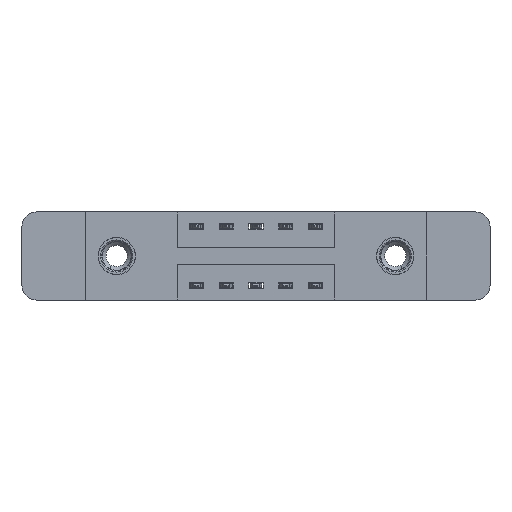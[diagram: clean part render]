
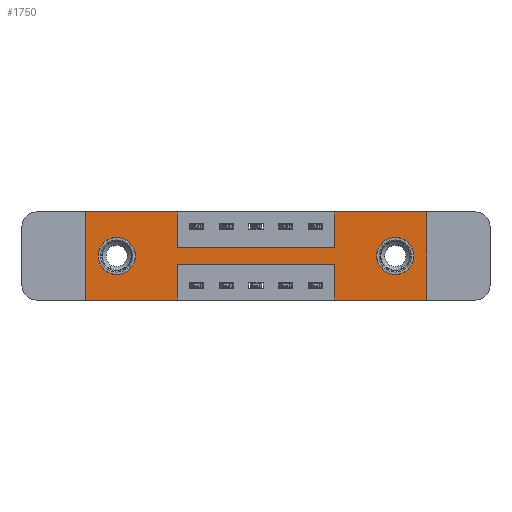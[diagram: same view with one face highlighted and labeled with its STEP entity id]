
A CAD part, front view. The second image highlights one B-rep face of the part: STEP entity #1750.
In plain terms, the highlighted planar face has unit normal (0, -1, 0).
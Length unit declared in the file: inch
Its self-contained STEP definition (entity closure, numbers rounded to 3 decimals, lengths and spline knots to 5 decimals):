
#126 = CIRCLE ( 'NONE', #325, 0.078 ) ;
#208 = DIRECTION ( 'NONE',  ( 0., 0., -1. ) ) ;
#225 = CARTESIAN_POINT ( 'NONE',  ( 0.3875, 0., -0.37 ) ) ;
#251 = DIRECTION ( 'NONE',  ( 0., 1., 0. ) ) ;
#325 = AXIS2_PLACEMENT_3D ( 'NONE', #10204, #13440, #1972 ) ;
#405 = VERTEX_POINT ( 'NONE', #8320 ) ;
#423 = ORIENTED_EDGE ( 'NONE', *, *, #3443, .T. ) ;
#483 = CARTESIAN_POINT ( 'NONE',  ( 0., 0., -0.37 ) ) ;
#484 = LINE ( 'NONE', #9128, #3106 ) ;
#711 = FACE_BOUND ( 'NONE', #7134, .T. ) ;
#802 = VERTEX_POINT ( 'NONE', #5080 ) ;
#832 = DIRECTION ( 'NONE',  ( 0., 0., -1. ) ) ;
#887 = CARTESIAN_POINT ( 'NONE',  ( 0., 0., 0. ) ) ;
#985 = DIRECTION ( 'NONE',  ( -1., 0., 0. ) ) ;
#1118 = VERTEX_POINT ( 'NONE', #9401 ) ;
#1128 = EDGE_CURVE ( 'NONE', #8901, #7750, #3313, .T. ) ;
#1283 = CARTESIAN_POINT ( 'NONE',  ( 0.3875, 0., -0.15 ) ) ;
#1629 = DIRECTION ( 'NONE',  ( 0., 0., 1. ) ) ;
#1730 = CARTESIAN_POINT ( 'NONE',  ( 0.1325, 0., -0.185 ) ) ;
#1750 = ADVANCED_FACE ( 'NONE', ( #4308, #711, #3184 ), #10912, .T. ) ;
#1767 = VERTEX_POINT ( 'NONE', #9796 ) ;
#1933 = EDGE_CURVE ( 'NONE', #405, #2278, #11183, .T. ) ;
#1972 = DIRECTION ( 'NONE',  ( 0., 0., 1. ) ) ;
#1990 = EDGE_CURVE ( 'NONE', #1767, #405, #12183, .T. ) ;
#2102 = DIRECTION ( 'NONE',  ( 1., 0., 0. ) ) ;
#2123 = EDGE_CURVE ( 'NONE', #6096, #5259, #12951, .T. ) ;
#2132 = CARTESIAN_POINT ( 'NONE',  ( 1.3025, 0., -0.263 ) ) ;
#2149 = LINE ( 'NONE', #887, #3919 ) ;
#2196 = VERTEX_POINT ( 'NONE', #7878 ) ;
#2278 = VERTEX_POINT ( 'NONE', #12317 ) ;
#2410 = CARTESIAN_POINT ( 'NONE',  ( 1.3025, 0., -0.185 ) ) ;
#2442 = DIRECTION ( 'NONE',  ( 0., 0., -1. ) ) ;
#2500 = EDGE_CURVE ( 'NONE', #802, #11937, #4712, .T. ) ;
#2667 = ORIENTED_EDGE ( 'NONE', *, *, #8357, .T. ) ;
#2675 = LINE ( 'NONE', #8262, #5749 ) ;
#2708 = VERTEX_POINT ( 'NONE', #3699 ) ;
#2844 = CARTESIAN_POINT ( 'NONE',  ( 0., 0., -0.37 ) ) ;
#3106 = VECTOR ( 'NONE', #11292, 39.37008 ) ;
#3184 = FACE_OUTER_BOUND ( 'NONE', #8724, .T. ) ;
#3188 = CARTESIAN_POINT ( 'NONE',  ( 0.3875, 0., 0. ) ) ;
#3302 = CARTESIAN_POINT ( 'NONE',  ( 0., 0., 0. ) ) ;
#3305 = DIRECTION ( 'NONE',  ( 0., 1., 0. ) ) ;
#3313 = LINE ( 'NONE', #3188, #6342 ) ;
#3443 = EDGE_CURVE ( 'NONE', #1118, #6664, #11835, .T. ) ;
#3459 = DIRECTION ( 'NONE',  ( 1., 0., 0. ) ) ;
#3621 = CARTESIAN_POINT ( 'NONE',  ( 0.1325, 0., -0.107 ) ) ;
#3652 = ORIENTED_EDGE ( 'NONE', *, *, #9171, .F. ) ;
#3699 = CARTESIAN_POINT ( 'NONE',  ( 1.0475, 0., -0.15 ) ) ;
#3751 = DIRECTION ( 'NONE',  ( 0., 0., 1. ) ) ;
#3919 = VECTOR ( 'NONE', #8163, 39.37008 ) ;
#4001 = ORIENTED_EDGE ( 'NONE', *, *, #1990, .F. ) ;
#4080 = VECTOR ( 'NONE', #3459, 39.37008 ) ;
#4308 = FACE_BOUND ( 'NONE', #11568, .T. ) ;
#4712 = LINE ( 'NONE', #3302, #11293 ) ;
#5011 = ORIENTED_EDGE ( 'NONE', *, *, #10540, .F. ) ;
#5080 = CARTESIAN_POINT ( 'NONE',  ( 1.0475, 0., 0. ) ) ;
#5205 = ORIENTED_EDGE ( 'NONE', *, *, #2123, .T. ) ;
#5259 = VERTEX_POINT ( 'NONE', #11602 ) ;
#5445 = EDGE_CURVE ( 'NONE', #11937, #13193, #2675, .T. ) ;
#5688 = ORIENTED_EDGE ( 'NONE', *, *, #2500, .F. ) ;
#5729 = ORIENTED_EDGE ( 'NONE', *, *, #5445, .F. ) ;
#5749 = VECTOR ( 'NONE', #832, 39.37008 ) ;
#5943 = DIRECTION ( 'NONE',  ( 0., 1., 0. ) ) ;
#6096 = VERTEX_POINT ( 'NONE', #3621 ) ;
#6342 = VECTOR ( 'NONE', #208, 39.37008 ) ;
#6360 = AXIS2_PLACEMENT_3D ( 'NONE', #2410, #251, #11756 ) ;
#6361 = LINE ( 'NONE', #10067, #10903 ) ;
#6664 = VERTEX_POINT ( 'NONE', #2132 ) ;
#6930 = DIRECTION ( 'NONE',  ( 0., 0., 1. ) ) ;
#7134 = EDGE_LOOP ( 'NONE', ( #5205, #10521 ) ) ;
#7172 = VECTOR ( 'NONE', #10308, 39.37008 ) ;
#7341 = LINE ( 'NONE', #9085, #10072 ) ;
#7512 = LINE ( 'NONE', #2844, #7172 ) ;
#7750 = VERTEX_POINT ( 'NONE', #8631 ) ;
#7878 = CARTESIAN_POINT ( 'NONE',  ( 1.0475, 0., -0.37 ) ) ;
#7981 = ORIENTED_EDGE ( 'NONE', *, *, #10708, .F. ) ;
#8044 = VECTOR ( 'NONE', #1629, 39.37008 ) ;
#8163 = DIRECTION ( 'NONE',  ( 1., 0., 0. ) ) ;
#8262 = CARTESIAN_POINT ( 'NONE',  ( 1.435, 0., 0. ) ) ;
#8320 = CARTESIAN_POINT ( 'NONE',  ( 0.3875, 0., -0.37 ) ) ;
#8357 = EDGE_CURVE ( 'NONE', #6664, #1118, #8941, .T. ) ;
#8616 = DIRECTION ( 'NONE',  ( 0., 0., -1. ) ) ;
#8631 = CARTESIAN_POINT ( 'NONE',  ( 0.3875, 0., -0.15 ) ) ;
#8724 = EDGE_LOOP ( 'NONE', ( #4001, #3652, #11326, #9885, #5729, #5688, #13030, #11518, #12730, #7981, #5011, #8848 ) ) ;
#8848 = ORIENTED_EDGE ( 'NONE', *, *, #1933, .F. ) ;
#8853 = CARTESIAN_POINT ( 'NONE',  ( 1.435, 0., -0.37 ) ) ;
#8901 = VERTEX_POINT ( 'NONE', #11196 ) ;
#8941 = CIRCLE ( 'NONE', #6360, 0.078 ) ;
#8994 = AXIS2_PLACEMENT_3D ( 'NONE', #1730, #5943, #6930 ) ;
#9085 = CARTESIAN_POINT ( 'NONE',  ( 1.0475, 0., -0.37 ) ) ;
#9128 = CARTESIAN_POINT ( 'NONE',  ( 1.0475, 0., 0. ) ) ;
#9132 = DIRECTION ( 'NONE',  ( -1., 0., 0. ) ) ;
#9171 = EDGE_CURVE ( 'NONE', #12392, #1767, #6361, .T. ) ;
#9307 = VERTEX_POINT ( 'NONE', #10023 ) ;
#9336 = VECTOR ( 'NONE', #8616, 39.37008 ) ;
#9401 = CARTESIAN_POINT ( 'NONE',  ( 1.3025, 0., -0.107 ) ) ;
#9555 = CARTESIAN_POINT ( 'NONE',  ( 1.3025, 0., -0.185 ) ) ;
#9714 = DIRECTION ( 'NONE',  ( 0., -1., 0. ) ) ;
#9796 = CARTESIAN_POINT ( 'NONE',  ( 0.3875, 0., -0.22 ) ) ;
#9831 = LINE ( 'NONE', #13178, #8044 ) ;
#9885 = ORIENTED_EDGE ( 'NONE', *, *, #10859, .F. ) ;
#9975 = EDGE_CURVE ( 'NONE', #7750, #2708, #10961, .T. ) ;
#10023 = CARTESIAN_POINT ( 'NONE',  ( 0., 0., 0. ) ) ;
#10067 = CARTESIAN_POINT ( 'NONE',  ( 0.3875, 0., -0.22 ) ) ;
#10072 = VECTOR ( 'NONE', #3751, 39.37008 ) ;
#10204 = CARTESIAN_POINT ( 'NONE',  ( 0.1325, 0., -0.185 ) ) ;
#10223 = EDGE_CURVE ( 'NONE', #2196, #12392, #7341, .T. ) ;
#10279 = CARTESIAN_POINT ( 'NONE',  ( 0., 0., -0.37 ) ) ;
#10308 = DIRECTION ( 'NONE',  ( -1., 0., 0. ) ) ;
#10521 = ORIENTED_EDGE ( 'NONE', *, *, #12513, .T. ) ;
#10540 = EDGE_CURVE ( 'NONE', #2278, #9307, #9831, .T. ) ;
#10708 = EDGE_CURVE ( 'NONE', #9307, #8901, #2149, .T. ) ;
#10716 = DIRECTION ( 'NONE',  ( 0., 0., -1. ) ) ;
#10844 = CARTESIAN_POINT ( 'NONE',  ( 1.0475, 0., -0.22 ) ) ;
#10859 = EDGE_CURVE ( 'NONE', #13193, #2196, #7512, .T. ) ;
#10903 = VECTOR ( 'NONE', #985, 39.37008 ) ;
#10912 = PLANE ( 'NONE',  #12642 ) ;
#10961 = LINE ( 'NONE', #1283, #4080 ) ;
#10995 = VECTOR ( 'NONE', #9132, 39.37008 ) ;
#11183 = LINE ( 'NONE', #10279, #10995 ) ;
#11196 = CARTESIAN_POINT ( 'NONE',  ( 0.3875, 0., 0. ) ) ;
#11292 = DIRECTION ( 'NONE',  ( 0., 0., 1. ) ) ;
#11293 = VECTOR ( 'NONE', #2102, 39.37008 ) ;
#11326 = ORIENTED_EDGE ( 'NONE', *, *, #10223, .F. ) ;
#11344 = CARTESIAN_POINT ( 'NONE',  ( 1.435, 0., 0. ) ) ;
#11518 = ORIENTED_EDGE ( 'NONE', *, *, #9975, .F. ) ;
#11568 = EDGE_LOOP ( 'NONE', ( #423, #2667 ) ) ;
#11602 = CARTESIAN_POINT ( 'NONE',  ( 0.1325, 0., -0.263 ) ) ;
#11756 = DIRECTION ( 'NONE',  ( 0., 0., -1. ) ) ;
#11835 = CIRCLE ( 'NONE', #11897, 0.078 ) ;
#11897 = AXIS2_PLACEMENT_3D ( 'NONE', #9555, #3305, #10716 ) ;
#11937 = VERTEX_POINT ( 'NONE', #11344 ) ;
#11942 = EDGE_CURVE ( 'NONE', #2708, #802, #484, .T. ) ;
#12183 = LINE ( 'NONE', #225, #9336 ) ;
#12317 = CARTESIAN_POINT ( 'NONE',  ( 0., 0., -0.37 ) ) ;
#12392 = VERTEX_POINT ( 'NONE', #10844 ) ;
#12513 = EDGE_CURVE ( 'NONE', #5259, #6096, #126, .T. ) ;
#12642 = AXIS2_PLACEMENT_3D ( 'NONE', #483, #9714, #2442 ) ;
#12730 = ORIENTED_EDGE ( 'NONE', *, *, #1128, .F. ) ;
#12951 = CIRCLE ( 'NONE', #8994, 0.078 ) ;
#13030 = ORIENTED_EDGE ( 'NONE', *, *, #11942, .F. ) ;
#13178 = CARTESIAN_POINT ( 'NONE',  ( 0., 0., 0. ) ) ;
#13193 = VERTEX_POINT ( 'NONE', #8853 ) ;
#13440 = DIRECTION ( 'NONE',  ( 0., 1., 0. ) ) ;
